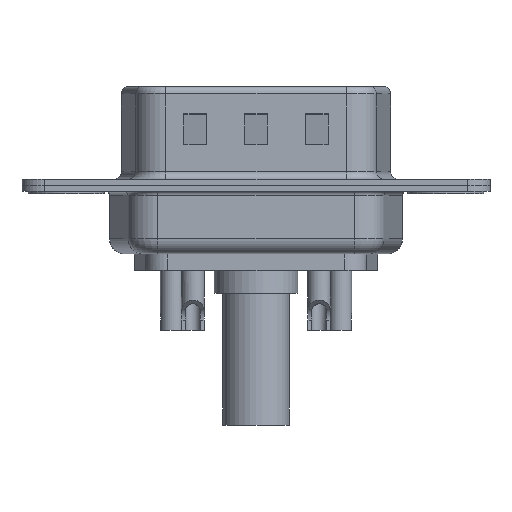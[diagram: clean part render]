
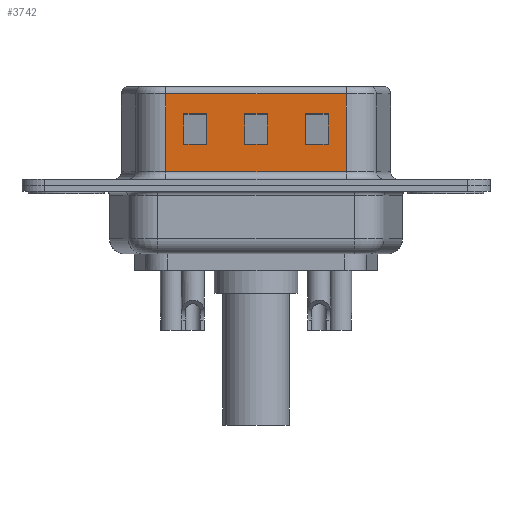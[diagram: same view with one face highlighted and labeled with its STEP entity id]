
A CAD part, front view. The second image highlights one B-rep face of the part: STEP entity #3742.
In plain terms, the highlighted planar face has unit normal (0, -1, 0).
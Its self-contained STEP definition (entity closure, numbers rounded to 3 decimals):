
#70 = VERTEX_POINT ( 'NONE', #559 ) ;
#160 = CARTESIAN_POINT ( 'NONE',  ( 7.75, -4.58, 2.705 ) ) ;
#434 = CARTESIAN_POINT ( 'NONE',  ( 18.45, -4.58, 6.52 ) ) ;
#436 = ORIENTED_EDGE ( 'NONE', *, *, #10728, .T. ) ;
#480 = DIRECTION ( 'NONE',  ( -1., 0., 0. ) ) ;
#487 = CARTESIAN_POINT ( 'NONE',  ( 18.45, -4.58, 6.52 ) ) ;
#559 = CARTESIAN_POINT ( 'NONE',  ( 15.75, -4.58, 2.705 ) ) ;
#754 = EDGE_CURVE ( 'NONE', #2137, #5916, #6359, .T. ) ;
#775 = LINE ( 'NONE', #5583, #5378 ) ;
#935 = EDGE_CURVE ( 'NONE', #9391, #1912, #5568, .T. ) ;
#960 = LINE ( 'NONE', #2717, #9028 ) ;
#976 = DIRECTION ( 'NONE',  ( 1., 0., 0. ) ) ;
#1085 = PLANE ( 'NONE',  #10195 ) ;
#1292 = CARTESIAN_POINT ( 'NONE',  ( 6.55, -4.58, 6.02 ) ) ;
#1396 = LINE ( 'NONE', #9054, #8847 ) ;
#1633 = EDGE_CURVE ( 'NONE', #8750, #2137, #1688, .T. ) ;
#1688 = LINE ( 'NONE', #12163, #11705 ) ;
#1696 = DIRECTION ( 'NONE',  ( 0., 1., 0. ) ) ;
#1742 = DIRECTION ( 'NONE',  ( 0., 0., 1. ) ) ;
#1744 = DIRECTION ( 'NONE',  ( 0., 0., -1. ) ) ;
#1803 = CARTESIAN_POINT ( 'NONE',  ( 7.75, -4.58, 4.705 ) ) ;
#1830 = ORIENTED_EDGE ( 'NONE', *, *, #12018, .T. ) ;
#1912 = VERTEX_POINT ( 'NONE', #1803 ) ;
#1976 = CARTESIAN_POINT ( 'NONE',  ( 6.55, -4.58, 6.52 ) ) ;
#2089 = LINE ( 'NONE', #9069, #9860 ) ;
#2137 = VERTEX_POINT ( 'NONE', #10546 ) ;
#2238 = EDGE_CURVE ( 'NONE', #1912, #6053, #775, .T. ) ;
#2264 = VECTOR ( 'NONE', #9569, 1000. ) ;
#2427 = DIRECTION ( 'NONE',  ( 0., 0., -1. ) ) ;
#2559 = LINE ( 'NONE', #5726, #12243 ) ;
#2563 = CARTESIAN_POINT ( 'NONE',  ( 13.25, -4.58, 2.705 ) ) ;
#2566 = ORIENTED_EDGE ( 'NONE', *, *, #8821, .T. ) ;
#2593 = EDGE_LOOP ( 'NONE', ( #11266, #9709, #9164, #10414 ) ) ;
#2614 = LINE ( 'NONE', #2994, #10061 ) ;
#2627 = LINE ( 'NONE', #7114, #7822 ) ;
#2679 = CARTESIAN_POINT ( 'NONE',  ( 15.75, -4.58, 4.705 ) ) ;
#2717 = CARTESIAN_POINT ( 'NONE',  ( 17.25, -4.58, 6.52 ) ) ;
#2859 = EDGE_CURVE ( 'NONE', #5082, #4073, #11818, .T. ) ;
#2943 = VECTOR ( 'NONE', #6550, 1000. ) ;
#2994 = CARTESIAN_POINT ( 'NONE',  ( 22.45, -4.58, 4.705 ) ) ;
#3039 = FACE_OUTER_BOUND ( 'NONE', #5918, .T. ) ;
#3742 = ADVANCED_FACE ( 'NONE', ( #8216, #5972, #5663, #3039 ), #1085, .F. ) ;
#4045 = EDGE_CURVE ( 'NONE', #5916, #10001, #2559, .T. ) ;
#4072 = VECTOR ( 'NONE', #480, 1000. ) ;
#4073 = VERTEX_POINT ( 'NONE', #8946 ) ;
#4398 = LINE ( 'NONE', #9153, #6108 ) ;
#4765 = DIRECTION ( 'NONE',  ( 1., 0., 0. ) ) ;
#4780 = DIRECTION ( 'NONE',  ( 0., 0., 1. ) ) ;
#5049 = DIRECTION ( 'NONE',  ( 1., 0., 0. ) ) ;
#5082 = VERTEX_POINT ( 'NONE', #7621 ) ;
#5378 = VECTOR ( 'NONE', #4765, 1000. ) ;
#5437 = CARTESIAN_POINT ( 'NONE',  ( 7.75, -4.58, 6.52 ) ) ;
#5568 = LINE ( 'NONE', #5437, #2943 ) ;
#5583 = CARTESIAN_POINT ( 'NONE',  ( 14.45, -4.58, 4.705 ) ) ;
#5616 = EDGE_CURVE ( 'NONE', #5082, #9820, #11756, .T. ) ;
#5631 = VERTEX_POINT ( 'NONE', #6718 ) ;
#5663 = FACE_BOUND ( 'NONE', #6987, .T. ) ;
#5726 = CARTESIAN_POINT ( 'NONE',  ( 13.25, -4.58, 6.52 ) ) ;
#5916 = VERTEX_POINT ( 'NONE', #7578 ) ;
#5918 = EDGE_LOOP ( 'NONE', ( #7847, #10662, #7712, #11078 ) ) ;
#5972 = FACE_BOUND ( 'NONE', #10277, .T. ) ;
#5990 = DIRECTION ( 'NONE',  ( 0., 0., -1. ) ) ;
#5993 = CARTESIAN_POINT ( 'NONE',  ( 18.45, -4.58, 6.02 ) ) ;
#6053 = VERTEX_POINT ( 'NONE', #6834 ) ;
#6108 = VECTOR ( 'NONE', #11081, 1000. ) ;
#6202 = DIRECTION ( 'NONE',  ( 0., 0., -1. ) ) ;
#6359 = LINE ( 'NONE', #9511, #7678 ) ;
#6550 = DIRECTION ( 'NONE',  ( 0., 0., 1. ) ) ;
#6613 = VERTEX_POINT ( 'NONE', #7894 ) ;
#6718 = CARTESIAN_POINT ( 'NONE',  ( 17.25, -4.58, 2.705 ) ) ;
#6834 = CARTESIAN_POINT ( 'NONE',  ( 9.25, -4.58, 4.705 ) ) ;
#6902 = EDGE_CURVE ( 'NONE', #11761, #5631, #960, .T. ) ;
#6987 = EDGE_LOOP ( 'NONE', ( #8290, #9280, #11839, #11766 ) ) ;
#7114 = CARTESIAN_POINT ( 'NONE',  ( 18.45, -4.58, 0.9 ) ) ;
#7139 = DIRECTION ( 'NONE',  ( -1., 0., 0. ) ) ;
#7532 = EDGE_CURVE ( 'NONE', #6613, #4073, #2627, .T. ) ;
#7551 = DIRECTION ( 'NONE',  ( 1., 0., 0. ) ) ;
#7578 = CARTESIAN_POINT ( 'NONE',  ( 13.25, -4.58, 4.705 ) ) ;
#7621 = CARTESIAN_POINT ( 'NONE',  ( 18.45, -4.58, 6.02 ) ) ;
#7653 = VECTOR ( 'NONE', #1744, 1000. ) ;
#7678 = VECTOR ( 'NONE', #7551, 1000. ) ;
#7712 = ORIENTED_EDGE ( 'NONE', *, *, #9003, .T. ) ;
#7822 = VECTOR ( 'NONE', #5049, 1000. ) ;
#7840 = CARTESIAN_POINT ( 'NONE',  ( 22.45, -4.58, 2.705 ) ) ;
#7847 = ORIENTED_EDGE ( 'NONE', *, *, #2859, .F. ) ;
#7894 = CARTESIAN_POINT ( 'NONE',  ( 6.55, -4.58, 0.9 ) ) ;
#8216 = FACE_BOUND ( 'NONE', #2593, .T. ) ;
#8290 = ORIENTED_EDGE ( 'NONE', *, *, #754, .T. ) ;
#8429 = CARTESIAN_POINT ( 'NONE',  ( 17.25, -4.58, 4.705 ) ) ;
#8578 = CARTESIAN_POINT ( 'NONE',  ( 15.75, -4.58, 6.52 ) ) ;
#8619 = DIRECTION ( 'NONE',  ( -1., 0., 0. ) ) ;
#8750 = VERTEX_POINT ( 'NONE', #10108 ) ;
#8821 = EDGE_CURVE ( 'NONE', #5631, #70, #9151, .T. ) ;
#8847 = VECTOR ( 'NONE', #7139, 1000. ) ;
#8946 = CARTESIAN_POINT ( 'NONE',  ( 18.45, -4.58, 0.9 ) ) ;
#8968 = VECTOR ( 'NONE', #5990, 1000. ) ;
#9003 = EDGE_CURVE ( 'NONE', #9820, #6613, #12438, .T. ) ;
#9028 = VECTOR ( 'NONE', #2427, 1000. ) ;
#9054 = CARTESIAN_POINT ( 'NONE',  ( 14.45, -4.58, 2.705 ) ) ;
#9068 = ORIENTED_EDGE ( 'NONE', *, *, #6902, .T. ) ;
#9069 = CARTESIAN_POINT ( 'NONE',  ( 9.25, -4.58, 6.52 ) ) ;
#9151 = LINE ( 'NONE', #7840, #11699 ) ;
#9153 = CARTESIAN_POINT ( 'NONE',  ( 18.45, -4.58, 2.705 ) ) ;
#9164 = ORIENTED_EDGE ( 'NONE', *, *, #935, .T. ) ;
#9275 = CARTESIAN_POINT ( 'NONE',  ( 9.25, -4.58, 2.705 ) ) ;
#9280 = ORIENTED_EDGE ( 'NONE', *, *, #4045, .T. ) ;
#9391 = VERTEX_POINT ( 'NONE', #160 ) ;
#9511 = CARTESIAN_POINT ( 'NONE',  ( 18.45, -4.58, 4.705 ) ) ;
#9569 = DIRECTION ( 'NONE',  ( 0., 0., 1. ) ) ;
#9709 = ORIENTED_EDGE ( 'NONE', *, *, #12204, .T. ) ;
#9820 = VERTEX_POINT ( 'NONE', #1292 ) ;
#9860 = VECTOR ( 'NONE', #6202, 1000. ) ;
#10001 = VERTEX_POINT ( 'NONE', #2563 ) ;
#10023 = LINE ( 'NONE', #8578, #2264 ) ;
#10061 = VECTOR ( 'NONE', #976, 1000. ) ;
#10108 = CARTESIAN_POINT ( 'NONE',  ( 11.75, -4.58, 2.705 ) ) ;
#10195 = AXIS2_PLACEMENT_3D ( 'NONE', #487, #1696, #1742 ) ;
#10277 = EDGE_LOOP ( 'NONE', ( #9068, #2566, #436, #1830 ) ) ;
#10414 = ORIENTED_EDGE ( 'NONE', *, *, #2238, .T. ) ;
#10546 = CARTESIAN_POINT ( 'NONE',  ( 11.75, -4.58, 4.705 ) ) ;
#10662 = ORIENTED_EDGE ( 'NONE', *, *, #5616, .T. ) ;
#10701 = VERTEX_POINT ( 'NONE', #2679 ) ;
#10728 = EDGE_CURVE ( 'NONE', #70, #10701, #10023, .T. ) ;
#11078 = ORIENTED_EDGE ( 'NONE', *, *, #7532, .T. ) ;
#11081 = DIRECTION ( 'NONE',  ( -1., 0., 0. ) ) ;
#11266 = ORIENTED_EDGE ( 'NONE', *, *, #11557, .T. ) ;
#11557 = EDGE_CURVE ( 'NONE', #6053, #11690, #2089, .T. ) ;
#11611 = EDGE_CURVE ( 'NONE', #10001, #8750, #4398, .T. ) ;
#11690 = VERTEX_POINT ( 'NONE', #9275 ) ;
#11699 = VECTOR ( 'NONE', #8619, 1000. ) ;
#11705 = VECTOR ( 'NONE', #4780, 1000. ) ;
#11756 = LINE ( 'NONE', #5993, #4072 ) ;
#11761 = VERTEX_POINT ( 'NONE', #8429 ) ;
#11766 = ORIENTED_EDGE ( 'NONE', *, *, #1633, .T. ) ;
#11818 = LINE ( 'NONE', #434, #8968 ) ;
#11839 = ORIENTED_EDGE ( 'NONE', *, *, #11611, .T. ) ;
#11931 = DIRECTION ( 'NONE',  ( 0., 0., -1. ) ) ;
#12018 = EDGE_CURVE ( 'NONE', #10701, #11761, #2614, .T. ) ;
#12163 = CARTESIAN_POINT ( 'NONE',  ( 11.75, -4.58, 6.52 ) ) ;
#12204 = EDGE_CURVE ( 'NONE', #11690, #9391, #1396, .T. ) ;
#12243 = VECTOR ( 'NONE', #11931, 1000. ) ;
#12438 = LINE ( 'NONE', #1976, #7653 ) ;
